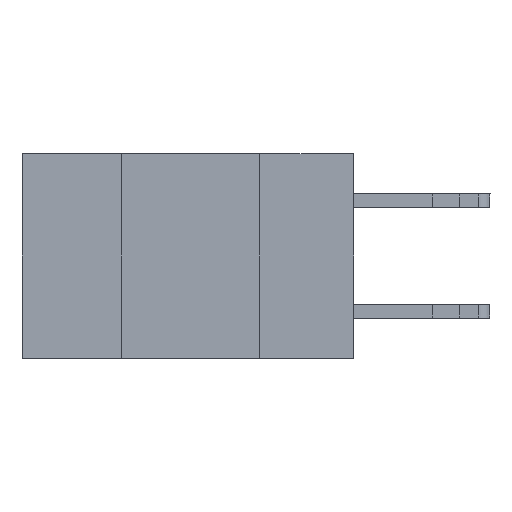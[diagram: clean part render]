
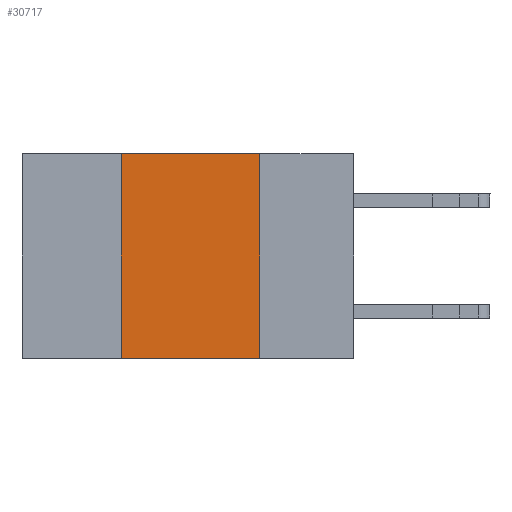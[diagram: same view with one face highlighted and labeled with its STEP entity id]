
A CAD part, left-side view. The second image highlights one B-rep face of the part: STEP entity #30717.
In plain terms, the highlighted planar face has unit normal (-1, 0, 0).
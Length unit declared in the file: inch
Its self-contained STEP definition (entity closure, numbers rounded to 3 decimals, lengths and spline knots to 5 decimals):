
#1213 = DIRECTION ( 'NONE',  ( 0., 0., -1. ) ) ;
#1418 = EDGE_CURVE ( 'NONE', #2650, #21055, #15329, .T. ) ;
#2200 = PLANE ( 'NONE',  #34158 ) ;
#2650 = VERTEX_POINT ( 'NONE', #12744 ) ;
#4285 = CARTESIAN_POINT ( 'NONE',  ( 0., 0.42, 0. ) ) ;
#4993 = CARTESIAN_POINT ( 'NONE',  ( 0., 0.6, 0. ) ) ;
#5541 = EDGE_CURVE ( 'NONE', #6941, #2650, #18474, .T. ) ;
#6941 = VERTEX_POINT ( 'NONE', #7698 ) ;
#6965 = VERTEX_POINT ( 'NONE', #16613 ) ;
#7054 = ORIENTED_EDGE ( 'NONE', *, *, #35860, .T. ) ;
#7698 = CARTESIAN_POINT ( 'NONE',  ( 0., 0.42, 0. ) ) ;
#9205 = VECTOR ( 'NONE', #26972, 39.37008 ) ;
#10313 = LINE ( 'NONE', #24073, #11339 ) ;
#11339 = VECTOR ( 'NONE', #15881, 39.37008 ) ;
#12744 = CARTESIAN_POINT ( 'NONE',  ( 0., 0.17, 0. ) ) ;
#13078 = CARTESIAN_POINT ( 'NONE',  ( 0., 0.6, 0. ) ) ;
#13380 = ORIENTED_EDGE ( 'NONE', *, *, #1418, .F. ) ;
#14972 = CARTESIAN_POINT ( 'NONE',  ( 0., 0.17, 0. ) ) ;
#15135 = VECTOR ( 'NONE', #26841, 39.37008 ) ;
#15329 = LINE ( 'NONE', #14972, #28750 ) ;
#15881 = DIRECTION ( 'NONE',  ( 0., -1., 0. ) ) ;
#16231 = ORIENTED_EDGE ( 'NONE', *, *, #5541, .F. ) ;
#16613 = CARTESIAN_POINT ( 'NONE',  ( 0., 0.42, -0.37 ) ) ;
#17117 = EDGE_LOOP ( 'NONE', ( #13380, #16231, #33334, #7054 ) ) ;
#18474 = LINE ( 'NONE', #13078, #15135 ) ;
#19299 = DIRECTION ( 'NONE',  ( 0., 0., -1. ) ) ;
#21055 = VERTEX_POINT ( 'NONE', #24181 ) ;
#24073 = CARTESIAN_POINT ( 'NONE',  ( 0., 0.6, -0.37 ) ) ;
#24181 = CARTESIAN_POINT ( 'NONE',  ( 0., 0.17, -0.37 ) ) ;
#25425 = DIRECTION ( 'NONE',  ( 1., 0., 0. ) ) ;
#26841 = DIRECTION ( 'NONE',  ( 0., -1., 0. ) ) ;
#26972 = DIRECTION ( 'NONE',  ( 0., 0., 1. ) ) ;
#28750 = VECTOR ( 'NONE', #1213, 39.37008 ) ;
#30212 = EDGE_CURVE ( 'NONE', #6965, #6941, #32909, .T. ) ;
#30717 = ADVANCED_FACE ( 'NONE', ( #33601 ), #2200, .F. ) ;
#32909 = LINE ( 'NONE', #4285, #9205 ) ;
#33334 = ORIENTED_EDGE ( 'NONE', *, *, #30212, .F. ) ;
#33601 = FACE_OUTER_BOUND ( 'NONE', #17117, .T. ) ;
#34158 = AXIS2_PLACEMENT_3D ( 'NONE', #4993, #25425, #19299 ) ;
#35860 = EDGE_CURVE ( 'NONE', #6965, #21055, #10313, .T. ) ;
